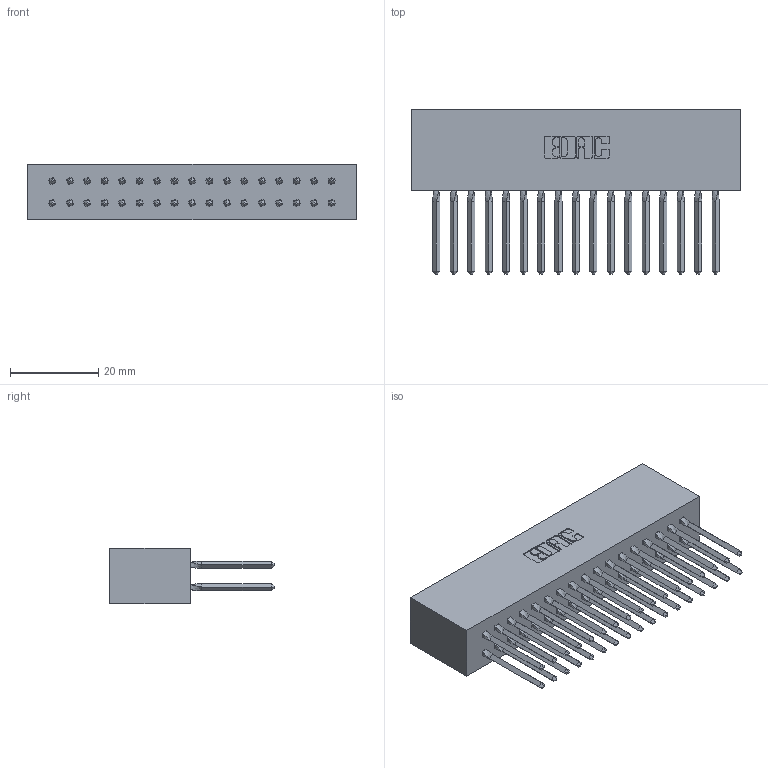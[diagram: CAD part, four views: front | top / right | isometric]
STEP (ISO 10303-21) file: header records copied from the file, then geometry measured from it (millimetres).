
FILE_DESCRIPTION (( 'STEP AP203' ), '1' );
FILE_NAME ('317-034-540-801.STEP', '2020-02-27T21:53:16', ( '' ), ( '' ), 'SwSTEP 2.0', 'SolidWorks 2016', '' );
FILE_SCHEMA (( 'CONFIG_CONTROL_DESIGN' ));
Length unit declared in the file: inch
Products named in the file (3): 317-034-540-801; 317-290-001_540; 317 Part_Lugless
Assembly tree (35 placements, depth 2):
  317-034-540-801
    317 Part_Lugless
    317-290-001_540  x34
Bounding box: 74.57 x 37.34 x 12.7 mm (x, y, z)
Volume: 13464.2 mm3; surface area: 19386.3 mm2
Topology: 35 solids, 35 shells, 3116 faces, 8637 edges, 5564 vertices
Faces by surface type: plane 2532, cylinder 448, bspline 136
Entity records: 27652 total; most frequent: CARTESIAN_POINT 5235, ORIENTED_EDGE 4734, DIRECTION 3945, EDGE_CURVE 2367, VECTOR 2119, LINE 2119, VERTEX_POINT 1571, AXIS2_PLACEMENT_3D 913
